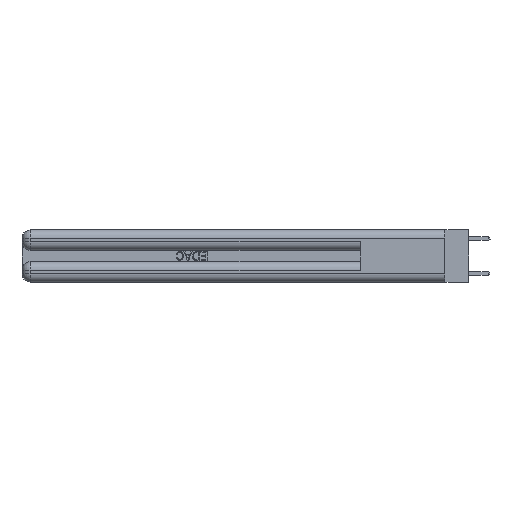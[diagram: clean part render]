
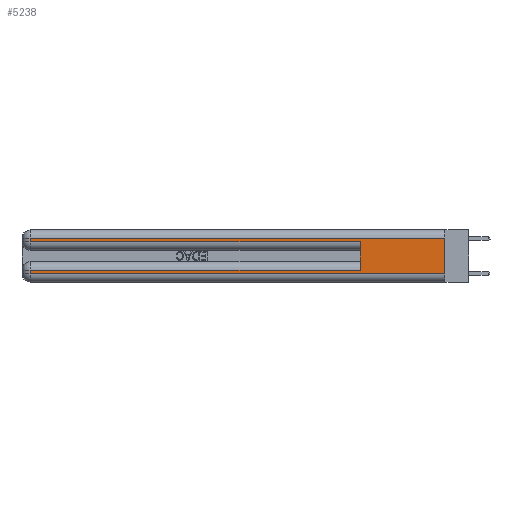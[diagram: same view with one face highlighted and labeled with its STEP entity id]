
A CAD part, left-side view. The second image highlights one B-rep face of the part: STEP entity #5238.
In plain terms, the highlighted planar face has unit normal (-1, 0, 0).
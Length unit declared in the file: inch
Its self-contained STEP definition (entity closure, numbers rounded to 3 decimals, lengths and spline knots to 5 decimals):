
#92 = VERTEX_POINT ( 'NONE', #23541 ) ;
#760 = CARTESIAN_POINT ( 'NONE',  ( 0., 0., 0.31 ) ) ;
#1379 = ORIENTED_EDGE ( 'NONE', *, *, #11069, .T. ) ;
#2045 = EDGE_CURVE ( 'NONE', #15117, #5162, #23926, .T. ) ;
#2417 = VECTOR ( 'NONE', #14466, 39.37008 ) ;
#3098 = VECTOR ( 'NONE', #14931, 39.37008 ) ;
#4044 = CARTESIAN_POINT ( 'NONE',  ( 0., 0., 0.37 ) ) ;
#5139 = PLANE ( 'NONE',  #11994 ) ;
#5162 = VERTEX_POINT ( 'NONE', #16101 ) ;
#5238 = ADVANCED_FACE ( 'NONE', ( #35804 ), #5139, .F. ) ;
#5464 = EDGE_CURVE ( 'NONE', #6973, #35622, #22687, .T. ) ;
#5755 = CARTESIAN_POINT ( 'NONE',  ( 0., 2.94, 0.31 ) ) ;
#6973 = VERTEX_POINT ( 'NONE', #5755 ) ;
#7182 = ORIENTED_EDGE ( 'NONE', *, *, #31941, .T. ) ;
#7322 = VECTOR ( 'NONE', #8808, 39.37008 ) ;
#8808 = DIRECTION ( 'NONE',  ( 0., 0., -1. ) ) ;
#9051 = VERTEX_POINT ( 'NONE', #28516 ) ;
#10225 = EDGE_CURVE ( 'NONE', #9051, #23440, #30957, .T. ) ;
#10597 = LINE ( 'NONE', #760, #3098 ) ;
#10670 = LINE ( 'NONE', #19263, #31040 ) ;
#10798 = DIRECTION ( 'NONE',  ( 1., 0., 0. ) ) ;
#11069 = EDGE_CURVE ( 'NONE', #92, #6973, #10597, .T. ) ;
#11170 = ORIENTED_EDGE ( 'NONE', *, *, #31433, .F. ) ;
#11187 = DIRECTION ( 'NONE',  ( 0., -1., 0. ) ) ;
#11274 = ORIENTED_EDGE ( 'NONE', *, *, #2045, .T. ) ;
#11994 = AXIS2_PLACEMENT_3D ( 'NONE', #27451, #10798, #30180 ) ;
#14466 = DIRECTION ( 'NONE',  ( 0., 1., 0. ) ) ;
#14707 = DIRECTION ( 'NONE',  ( 0., 0., -1. ) ) ;
#14931 = DIRECTION ( 'NONE',  ( 0., 1., 0. ) ) ;
#15117 = VERTEX_POINT ( 'NONE', #20586 ) ;
#15205 = VECTOR ( 'NONE', #18063, 39.37008 ) ;
#16101 = CARTESIAN_POINT ( 'NONE',  ( 0., 2.94, 0.085 ) ) ;
#16370 = ORIENTED_EDGE ( 'NONE', *, *, #10225, .T. ) ;
#17282 = ORIENTED_EDGE ( 'NONE', *, *, #5464, .T. ) ;
#18063 = DIRECTION ( 'NONE',  ( 0., 0., -1. ) ) ;
#18273 = CARTESIAN_POINT ( 'NONE',  ( 0., 0., 0.285 ) ) ;
#19202 = EDGE_LOOP ( 'NONE', ( #11170, #1379, #17282, #34442, #34763, #11274, #7182, #16370 ) ) ;
#19263 = CARTESIAN_POINT ( 'NONE',  ( 0., 0.6, 0.145 ) ) ;
#20586 = CARTESIAN_POINT ( 'NONE',  ( 0., 0.6, 0.085 ) ) ;
#21052 = DIRECTION ( 'NONE',  ( 0., -1., 0. ) ) ;
#22624 = LINE ( 'NONE', #4044, #15205 ) ;
#22687 = LINE ( 'NONE', #22891, #29091 ) ;
#22708 = CARTESIAN_POINT ( 'NONE',  ( 0., 0., 0.06 ) ) ;
#22891 = CARTESIAN_POINT ( 'NONE',  ( 0., 2.94, 0.37 ) ) ;
#23084 = LINE ( 'NONE', #25507, #7322 ) ;
#23440 = VERTEX_POINT ( 'NONE', #22708 ) ;
#23541 = CARTESIAN_POINT ( 'NONE',  ( 0., 0., 0.31 ) ) ;
#23649 = VECTOR ( 'NONE', #21052, 39.37008 ) ;
#23838 = VERTEX_POINT ( 'NONE', #35105 ) ;
#23926 = LINE ( 'NONE', #33657, #2417 ) ;
#24687 = DIRECTION ( 'NONE',  ( 0., 0., 1. ) ) ;
#25155 = VECTOR ( 'NONE', #11187, 39.37008 ) ;
#25507 = CARTESIAN_POINT ( 'NONE',  ( 0., 2.94, 0.37 ) ) ;
#26794 = EDGE_CURVE ( 'NONE', #35622, #23838, #31745, .T. ) ;
#27451 = CARTESIAN_POINT ( 'NONE',  ( 0., 0., 0.37 ) ) ;
#28516 = CARTESIAN_POINT ( 'NONE',  ( 0., 2.94, 0.06 ) ) ;
#29091 = VECTOR ( 'NONE', #14707, 39.37008 ) ;
#30180 = DIRECTION ( 'NONE',  ( 0., 0., -1. ) ) ;
#30957 = LINE ( 'NONE', #33227, #25155 ) ;
#31040 = VECTOR ( 'NONE', #24687, 39.37008 ) ;
#31433 = EDGE_CURVE ( 'NONE', #92, #23440, #22624, .T. ) ;
#31745 = LINE ( 'NONE', #18273, #23649 ) ;
#31941 = EDGE_CURVE ( 'NONE', #5162, #9051, #23084, .T. ) ;
#33191 = CARTESIAN_POINT ( 'NONE',  ( 0., 2.94, 0.285 ) ) ;
#33227 = CARTESIAN_POINT ( 'NONE',  ( 0., 0., 0.06 ) ) ;
#33574 = EDGE_CURVE ( 'NONE', #15117, #23838, #10670, .T. ) ;
#33657 = CARTESIAN_POINT ( 'NONE',  ( 0., 0., 0.085 ) ) ;
#34442 = ORIENTED_EDGE ( 'NONE', *, *, #26794, .T. ) ;
#34763 = ORIENTED_EDGE ( 'NONE', *, *, #33574, .F. ) ;
#35105 = CARTESIAN_POINT ( 'NONE',  ( 0., 0.6, 0.285 ) ) ;
#35622 = VERTEX_POINT ( 'NONE', #33191 ) ;
#35804 = FACE_OUTER_BOUND ( 'NONE', #19202, .T. ) ;
